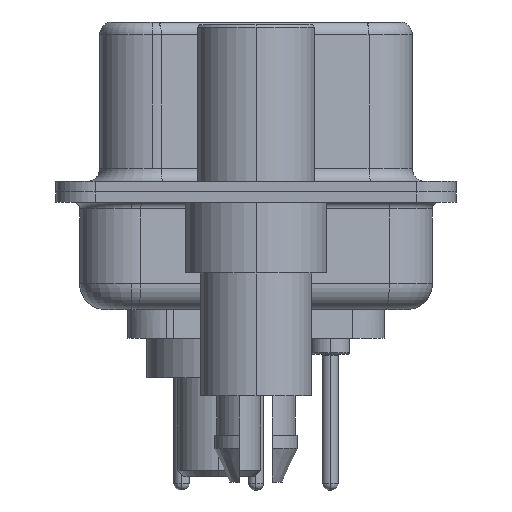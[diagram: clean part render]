
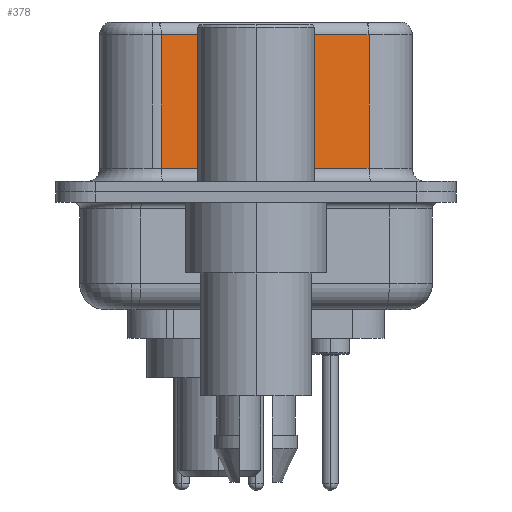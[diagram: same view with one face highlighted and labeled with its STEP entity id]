
A CAD part, left-side view. The second image highlights one B-rep face of the part: STEP entity #378.
In plain terms, the highlighted planar face has unit normal (-0.985, -0.174, 0).
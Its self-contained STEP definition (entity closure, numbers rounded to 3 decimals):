
#172 = CARTESIAN_POINT ( 'NONE',  ( 5.132, -4.322, 0.9 ) ) ;
#378 = ADVANCED_FACE ( 'NONE', ( #6877 ), #5314, .F. ) ;
#805 = ORIENTED_EDGE ( 'NONE', *, *, #15515, .T. ) ;
#1562 = DIRECTION ( 'NONE',  ( 0.985, 0.174, 0. ) ) ;
#1895 = CARTESIAN_POINT ( 'NONE',  ( 5.132, -4.322, 6.02 ) ) ;
#2059 = DIRECTION ( 'NONE',  ( -0.174, 0.985, 0. ) ) ;
#2523 = DIRECTION ( 'NONE',  ( 0.174, -0.985, 0. ) ) ;
#2775 = EDGE_CURVE ( 'NONE', #25107, #4040, #21084, .T. ) ;
#4040 = VERTEX_POINT ( 'NONE', #22709 ) ;
#4305 = CARTESIAN_POINT ( 'NONE',  ( 5.132, -4.322, 6.02 ) ) ;
#5276 = CARTESIAN_POINT ( 'NONE',  ( 5.132, -4.322, 6.52 ) ) ;
#5314 = PLANE ( 'NONE',  #8794 ) ;
#6179 = VERTEX_POINT ( 'NONE', #24866 ) ;
#6494 = LINE ( 'NONE', #12773, #24134 ) ;
#6877 = FACE_OUTER_BOUND ( 'NONE', #20735, .T. ) ;
#7721 = CARTESIAN_POINT ( 'NONE',  ( 3.73, 3.628, 6.02 ) ) ;
#8175 = DIRECTION ( 'NONE',  ( 0., 0., -1. ) ) ;
#8564 = LINE ( 'NONE', #172, #13936 ) ;
#8794 = AXIS2_PLACEMENT_3D ( 'NONE', #5276, #1562, #2059 ) ;
#8883 = VECTOR ( 'NONE', #20466, 1000. ) ;
#9032 = EDGE_CURVE ( 'NONE', #4040, #6179, #8564, .T. ) ;
#12041 = EDGE_CURVE ( 'NONE', #26366, #6179, #6494, .T. ) ;
#12773 = CARTESIAN_POINT ( 'NONE',  ( 5.132, -4.322, 6.52 ) ) ;
#13936 = VECTOR ( 'NONE', #2523, 1000. ) ;
#14396 = ORIENTED_EDGE ( 'NONE', *, *, #9032, .T. ) ;
#14952 = VECTOR ( 'NONE', #25693, 1000. ) ;
#15515 = EDGE_CURVE ( 'NONE', #26366, #25107, #27918, .T. ) ;
#16187 = ORIENTED_EDGE ( 'NONE', *, *, #2775, .T. ) ;
#20466 = DIRECTION ( 'NONE',  ( -0.174, 0.985, 0. ) ) ;
#20735 = EDGE_LOOP ( 'NONE', ( #27904, #805, #16187, #14396 ) ) ;
#21084 = LINE ( 'NONE', #22766, #14952 ) ;
#22709 = CARTESIAN_POINT ( 'NONE',  ( 3.73, 3.628, 0.9 ) ) ;
#22766 = CARTESIAN_POINT ( 'NONE',  ( 3.73, 3.628, 6.52 ) ) ;
#24134 = VECTOR ( 'NONE', #8175, 1000. ) ;
#24866 = CARTESIAN_POINT ( 'NONE',  ( 5.132, -4.322, 0.9 ) ) ;
#25107 = VERTEX_POINT ( 'NONE', #7721 ) ;
#25693 = DIRECTION ( 'NONE',  ( 0., 0., -1. ) ) ;
#26366 = VERTEX_POINT ( 'NONE', #4305 ) ;
#27904 = ORIENTED_EDGE ( 'NONE', *, *, #12041, .F. ) ;
#27918 = LINE ( 'NONE', #1895, #8883 ) ;
